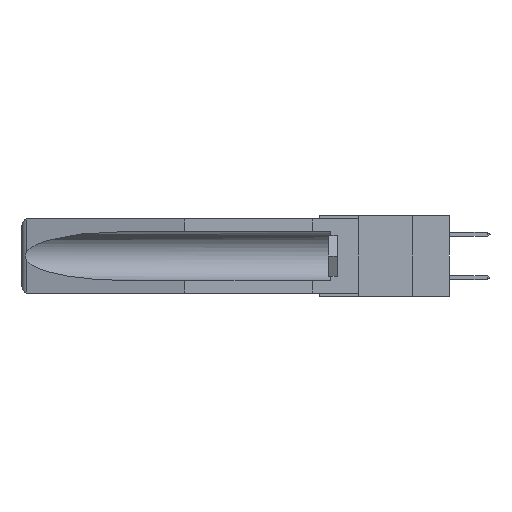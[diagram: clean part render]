
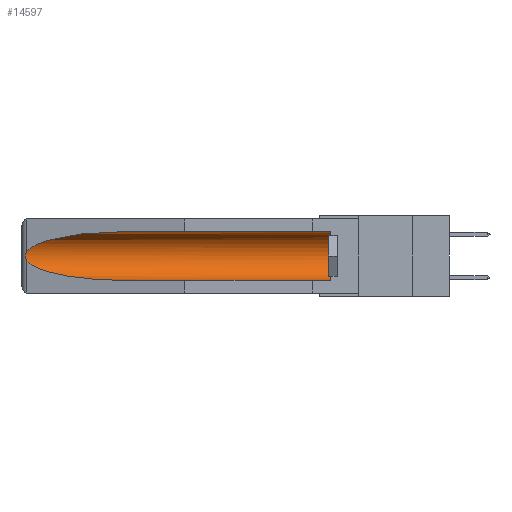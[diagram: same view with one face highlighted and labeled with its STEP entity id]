
A CAD part, left-side view. The second image highlights one B-rep face of the part: STEP entity #14597.
In plain terms, the highlighted cylindrical face has radius 2.857 mm (diameter 5.715 mm), a partial arc.
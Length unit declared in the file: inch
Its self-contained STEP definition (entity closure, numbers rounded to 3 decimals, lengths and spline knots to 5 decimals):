
#693 = LINE ( 'NONE', #17113, #27271 ) ;
#1307 =( BOUNDED_CURVE ( )  B_SPLINE_CURVE ( 3, ( #15915, #18253, #3026, #20632 ),
 .UNSPECIFIED., .F., .T. ) 
 B_SPLINE_CURVE_WITH_KNOTS ( ( 4, 4 ),
 ( 4.71239, 6.08839 ),
 .UNSPECIFIED. ) 
 CURVE ( )  GEOMETRIC_REPRESENTATION_ITEM ( )  RATIONAL_B_SPLINE_CURVE ( ( 1., 0.848, 0.848, 1. ) ) 
 REPRESENTATION_ITEM ( '' )  );
#1736 = DIRECTION ( 'NONE',  ( 0., 1., 0. ) ) ;
#1859 = EDGE_CURVE ( 'NONE', #2794, #22673, #9989, .T. ) ;
#2329 = CARTESIAN_POINT ( 'NONE',  ( 0.2675, 1.53308, -0.16763 ) ) ;
#2616 = CARTESIAN_POINT ( 'NONE',  ( 0.155, 0.126, -0.284 ) ) ;
#2650 = EDGE_CURVE ( 'NONE', #13586, #28081, #1307, .T. ) ;
#2794 = VERTEX_POINT ( 'NONE', #3246 ) ;
#3026 = CARTESIAN_POINT ( 'NONE',  ( 0.25451, 1.48313, -0.09465 ) ) ;
#3246 = CARTESIAN_POINT ( 'NONE',  ( 0.26537, 1.52718, -0.19328 ) ) ;
#4242 = CYLINDRICAL_SURFACE ( 'NONE', #21104, 0.1125 ) ;
#4527 = CARTESIAN_POINT ( 'NONE',  ( 0.155, -0.30754, -0.1715 ) ) ;
#4648 = DIRECTION ( 'NONE',  ( 0., 0., 1. ) ) ;
#5015 = CARTESIAN_POINT ( 'NONE',  ( 0.2673, 1.5327, -0.16383 ) ) ;
#5570 = CARTESIAN_POINT ( 'NONE',  ( 0.26537, 1.52718, -0.19328 ) ) ;
#6932 = CARTESIAN_POINT ( 'NONE',  ( 0.26537, 1.52718, -0.19328 ) ) ;
#7258 = ORIENTED_EDGE ( 'NONE', *, *, #2650, .T. ) ;
#7409 = CARTESIAN_POINT ( 'NONE',  ( 0.26537, 1.52718, -0.14972 ) ) ;
#7528 = ORIENTED_EDGE ( 'NONE', *, *, #16287, .T. ) ;
#8684 = ORIENTED_EDGE ( 'NONE', *, *, #1859, .T. ) ;
#9520 = CARTESIAN_POINT ( 'NONE',  ( 0.25451, 1.48313, -0.24835 ) ) ;
#9640 = DIRECTION ( 'NONE',  ( 0., 1., 0. ) ) ;
#9986 = CARTESIAN_POINT ( 'NONE',  ( 0.26654, 1.53092, -0.15636 ) ) ;
#9989 =( BOUNDED_CURVE ( )  B_SPLINE_CURVE ( 3, ( #6932, #9520, #16888, #12094 ),
 .UNSPECIFIED., .F., .F. ) 
 B_SPLINE_CURVE_WITH_KNOTS ( ( 4, 4 ),
 ( 0.1948, 1.5708 ),
 .UNSPECIFIED. ) 
 CURVE ( )  GEOMETRIC_REPRESENTATION_ITEM ( )  RATIONAL_B_SPLINE_CURVE ( ( 1., 0.848, 0.848, 1. ) ) 
 REPRESENTATION_ITEM ( '' )  );
#10533 = EDGE_CURVE ( 'NONE', #27649, #13586, #14874, .T. ) ;
#12094 = CARTESIAN_POINT ( 'NONE',  ( 0.155, 1.07973, -0.284 ) ) ;
#12681 = CARTESIAN_POINT ( 'NONE',  ( 0.26597, 1.5296, -0.19026 ) ) ;
#13080 = ORIENTED_EDGE ( 'NONE', *, *, #10533, .T. ) ;
#13142 = FACE_OUTER_BOUND ( 'NONE', #13992, .T. ) ;
#13586 = VERTEX_POINT ( 'NONE', #29008 ) ;
#13779 = CARTESIAN_POINT ( 'NONE',  ( 0.155, 0.126, -0.1715 ) ) ;
#13992 = EDGE_LOOP ( 'NONE', ( #7258, #14938, #8684, #29861, #7528, #13080 ) ) ;
#14010 = EDGE_CURVE ( 'NONE', #21824, #22673, #693, .T. ) ;
#14597 = ADVANCED_FACE ( 'NONE', ( #13142 ), #4242, .F. ) ;
#14635 = CIRCLE ( 'NONE', #33059, 0.1125 ) ;
#14874 = LINE ( 'NONE', #16719, #28590 ) ;
#14938 = ORIENTED_EDGE ( 'NONE', *, *, #29355, .T. ) ;
#15230 = CARTESIAN_POINT ( 'NONE',  ( 0.2675, 1.53308, -0.17534 ) ) ;
#15915 = CARTESIAN_POINT ( 'NONE',  ( 0.155, 1.07973, -0.059 ) ) ;
#16287 = EDGE_CURVE ( 'NONE', #21824, #27649, #14635, .T. ) ;
#16719 = CARTESIAN_POINT ( 'NONE',  ( 0.155, -0.30754, -0.059 ) ) ;
#16888 = CARTESIAN_POINT ( 'NONE',  ( 0.21114, 1.30732, -0.284 ) ) ;
#17113 = CARTESIAN_POINT ( 'NONE',  ( 0.155, -0.30754, -0.284 ) ) ;
#18253 = CARTESIAN_POINT ( 'NONE',  ( 0.21114, 1.30732, -0.059 ) ) ;
#18333 = CARTESIAN_POINT ( 'NONE',  ( 0.2673, 1.53269, -0.17917 ) ) ;
#20150 = CARTESIAN_POINT ( 'NONE',  ( 0.26655, 1.53094, -0.18657 ) ) ;
#20632 = CARTESIAN_POINT ( 'NONE',  ( 0.26537, 1.52718, -0.14972 ) ) ;
#21104 = AXIS2_PLACEMENT_3D ( 'NONE', #4527, #9640, #4648 ) ;
#21824 = VERTEX_POINT ( 'NONE', #2616 ) ;
#22573 = CARTESIAN_POINT ( 'NONE',  ( 0.155, 0.126, -0.059 ) ) ;
#22673 = VERTEX_POINT ( 'NONE', #23076 ) ;
#23076 = CARTESIAN_POINT ( 'NONE',  ( 0.155, 1.07973, -0.284 ) ) ;
#26394 = DIRECTION ( 'NONE',  ( 0., -1., 0. ) ) ;
#27271 = VECTOR ( 'NONE', #1736, 39.37008 ) ;
#27649 = VERTEX_POINT ( 'NONE', #22573 ) ;
#28076 = CARTESIAN_POINT ( 'NONE',  ( 0.26597, 1.52961, -0.15275 ) ) ;
#28081 = VERTEX_POINT ( 'NONE', #30234 ) ;
#28590 = VECTOR ( 'NONE', #29586, 39.37008 ) ;
#28771 = DIRECTION ( 'NONE',  ( 0., 0., 1. ) ) ;
#29008 = CARTESIAN_POINT ( 'NONE',  ( 0.155, 1.07973, -0.059 ) ) ;
#29355 = EDGE_CURVE ( 'NONE', #28081, #2794, #32036, .T. ) ;
#29586 = DIRECTION ( 'NONE',  ( 0., 1., 0. ) ) ;
#29861 = ORIENTED_EDGE ( 'NONE', *, *, #14010, .F. ) ;
#30234 = CARTESIAN_POINT ( 'NONE',  ( 0.26537, 1.52718, -0.14972 ) ) ;
#32036 = B_SPLINE_CURVE_WITH_KNOTS ( 'NONE', 3,
 ( #7409, #28076, #9986, #5015, #2329, #15230, #18333, #20150, #12681, #5570 ),
 .UNSPECIFIED., .F., .F.,
 ( 4, 2, 2, 2, 4 ),
 ( 0., 0.00029, 0.00058, 0.00087, 0.00117 ),
 .UNSPECIFIED. ) ;
#33059 = AXIS2_PLACEMENT_3D ( 'NONE', #13779, #26394, #28771 ) ;
